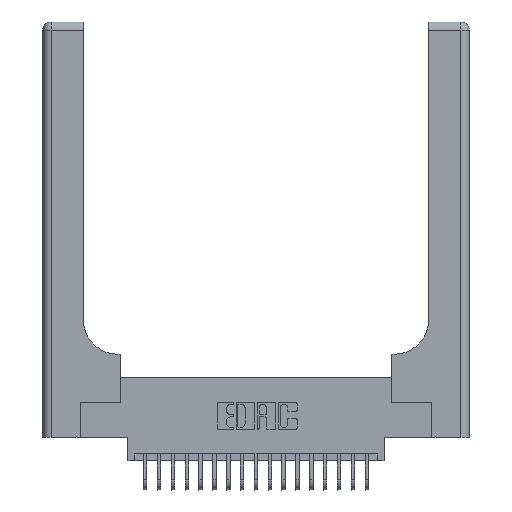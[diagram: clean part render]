
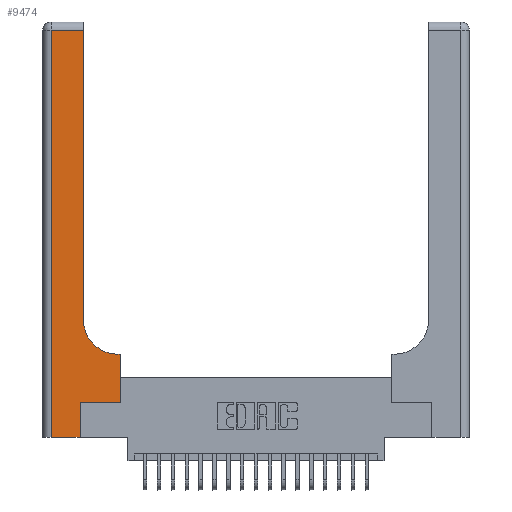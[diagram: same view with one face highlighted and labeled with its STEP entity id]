
A CAD part, top view. The second image highlights one B-rep face of the part: STEP entity #9474.
In plain terms, the highlighted planar face has unit normal (0, 0, 1).
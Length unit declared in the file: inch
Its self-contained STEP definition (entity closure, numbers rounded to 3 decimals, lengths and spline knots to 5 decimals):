
#308 = CARTESIAN_POINT ( 'NONE',  ( 0.2915, 2.94, 0.37 ) ) ;
#334 = EDGE_CURVE ( 'NONE', #5750, #17280, #9407, .T. ) ;
#569 = ORIENTED_EDGE ( 'NONE', *, *, #11895, .T. ) ;
#716 = VERTEX_POINT ( 'NONE', #4147 ) ;
#1633 = EDGE_CURVE ( 'NONE', #17578, #12482, #10521, .T. ) ;
#1995 = EDGE_CURVE ( 'NONE', #17280, #11936, #17637, .T. ) ;
#2028 = EDGE_CURVE ( 'NONE', #16891, #5750, #21936, .T. ) ;
#2461 = VECTOR ( 'NONE', #10708, 39.37008 ) ;
#2469 = DIRECTION ( 'NONE',  ( 0., 0., -1. ) ) ;
#2485 = FACE_OUTER_BOUND ( 'NONE', #15220, .T. ) ;
#2929 = DIRECTION ( 'NONE',  ( -1., 0., 0. ) ) ;
#3219 = ORIENTED_EDGE ( 'NONE', *, *, #6508, .T. ) ;
#3495 = DIRECTION ( 'NONE',  ( 0., 1., 0. ) ) ;
#4147 = CARTESIAN_POINT ( 'NONE',  ( 0.5415, 0.6, 0.37 ) ) ;
#4201 = VERTEX_POINT ( 'NONE', #15681 ) ;
#4488 = CARTESIAN_POINT ( 'NONE',  ( 0.5585, 0.6, 0.37 ) ) ;
#4505 = DIRECTION ( 'NONE',  ( 0., 0., -1. ) ) ;
#4705 = VECTOR ( 'NONE', #8935, 39.37008 ) ;
#5682 = ORIENTED_EDGE ( 'NONE', *, *, #12729, .T. ) ;
#5739 = CARTESIAN_POINT ( 'NONE',  ( 0.2915, 3., 0.37 ) ) ;
#5750 = VERTEX_POINT ( 'NONE', #8815 ) ;
#5785 = VECTOR ( 'NONE', #17432, 39.37008 ) ;
#6508 = EDGE_CURVE ( 'NONE', #4201, #16891, #22969, .T. ) ;
#6704 = EDGE_CURVE ( 'NONE', #18139, #4201, #22110, .T. ) ;
#6991 = LINE ( 'NONE', #21652, #4705 ) ;
#7233 = ORIENTED_EDGE ( 'NONE', *, *, #1633, .T. ) ;
#7691 = DIRECTION ( 'NONE',  ( 0., 1., 0. ) ) ;
#8089 = CARTESIAN_POINT ( 'NONE',  ( 0.5415, 0.85, 0.37 ) ) ;
#8344 = DIRECTION ( 'NONE',  ( -1., 0., 0. ) ) ;
#8368 = VECTOR ( 'NONE', #21697, 39.37008 ) ;
#8494 = CARTESIAN_POINT ( 'NONE',  ( 0.269, 0.25, 0.37 ) ) ;
#8815 = CARTESIAN_POINT ( 'NONE',  ( 0.269, 0.25, 0.37 ) ) ;
#8935 = DIRECTION ( 'NONE',  ( -1., 0., 0. ) ) ;
#9407 = LINE ( 'NONE', #8494, #11397 ) ;
#9474 = ADVANCED_FACE ( 'NONE', ( #2485 ), #10122, .F. ) ;
#9620 = CIRCLE ( 'NONE', #12505, 0.25 ) ;
#10122 = PLANE ( 'NONE',  #12341 ) ;
#10521 = LINE ( 'NONE', #5739, #23123 ) ;
#10660 = CARTESIAN_POINT ( 'NONE',  ( 0.2915, 0.85, 0.37 ) ) ;
#10708 = DIRECTION ( 'NONE',  ( 0., 1., 0. ) ) ;
#11397 = VECTOR ( 'NONE', #17369, 39.37008 ) ;
#11895 = EDGE_CURVE ( 'NONE', #716, #17578, #9620, .T. ) ;
#11936 = VERTEX_POINT ( 'NONE', #4488 ) ;
#12341 = AXIS2_PLACEMENT_3D ( 'NONE', #22911, #4505, #8344 ) ;
#12351 = CARTESIAN_POINT ( 'NONE',  ( 0.269, 0., 0.37 ) ) ;
#12482 = VERTEX_POINT ( 'NONE', #308 ) ;
#12505 = AXIS2_PLACEMENT_3D ( 'NONE', #8089, #2469, #19097 ) ;
#12521 = CARTESIAN_POINT ( 'NONE',  ( 0.5585, 0.25, 0.37 ) ) ;
#12606 = CARTESIAN_POINT ( 'NONE',  ( 0.06, 3., 0.37 ) ) ;
#12729 = EDGE_CURVE ( 'NONE', #12482, #18139, #6991, .T. ) ;
#12756 = VECTOR ( 'NONE', #3495, 39.37008 ) ;
#12934 = ORIENTED_EDGE ( 'NONE', *, *, #1995, .T. ) ;
#13511 = VECTOR ( 'NONE', #2929, 39.37008 ) ;
#14055 = ORIENTED_EDGE ( 'NONE', *, *, #2028, .T. ) ;
#14320 = CARTESIAN_POINT ( 'NONE',  ( 0., 0., 0.37 ) ) ;
#15220 = EDGE_LOOP ( 'NONE', ( #7233, #5682, #17072, #3219, #14055, #18015, #12934, #23096, #569 ) ) ;
#15681 = CARTESIAN_POINT ( 'NONE',  ( 0.06, 0., 0.37 ) ) ;
#16891 = VERTEX_POINT ( 'NONE', #12351 ) ;
#17072 = ORIENTED_EDGE ( 'NONE', *, *, #6704, .T. ) ;
#17280 = VERTEX_POINT ( 'NONE', #19053 ) ;
#17369 = DIRECTION ( 'NONE',  ( 1., 0., 0. ) ) ;
#17432 = DIRECTION ( 'NONE',  ( 0., -1., 0. ) ) ;
#17578 = VERTEX_POINT ( 'NONE', #10660 ) ;
#17637 = LINE ( 'NONE', #12521, #12756 ) ;
#18015 = ORIENTED_EDGE ( 'NONE', *, *, #334, .T. ) ;
#18123 = CARTESIAN_POINT ( 'NONE',  ( 0.269, 0., 0.37 ) ) ;
#18139 = VERTEX_POINT ( 'NONE', #23280 ) ;
#18366 = LINE ( 'NONE', #23191, #13511 ) ;
#19053 = CARTESIAN_POINT ( 'NONE',  ( 0.5585, 0.25, 0.37 ) ) ;
#19097 = DIRECTION ( 'NONE',  ( 1., 0., 0. ) ) ;
#21459 = EDGE_CURVE ( 'NONE', #11936, #716, #18366, .T. ) ;
#21652 = CARTESIAN_POINT ( 'NONE',  ( 0., 2.94, 0.37 ) ) ;
#21697 = DIRECTION ( 'NONE',  ( 1., 0., 0. ) ) ;
#21936 = LINE ( 'NONE', #18123, #2461 ) ;
#22110 = LINE ( 'NONE', #12606, #5785 ) ;
#22911 = CARTESIAN_POINT ( 'NONE',  ( 0., 3., 0.37 ) ) ;
#22969 = LINE ( 'NONE', #14320, #8368 ) ;
#23096 = ORIENTED_EDGE ( 'NONE', *, *, #21459, .T. ) ;
#23123 = VECTOR ( 'NONE', #7691, 39.37008 ) ;
#23191 = CARTESIAN_POINT ( 'NONE',  ( 0.2915, 0.6, 0.37 ) ) ;
#23280 = CARTESIAN_POINT ( 'NONE',  ( 0.06, 2.94, 0.37 ) ) ;
